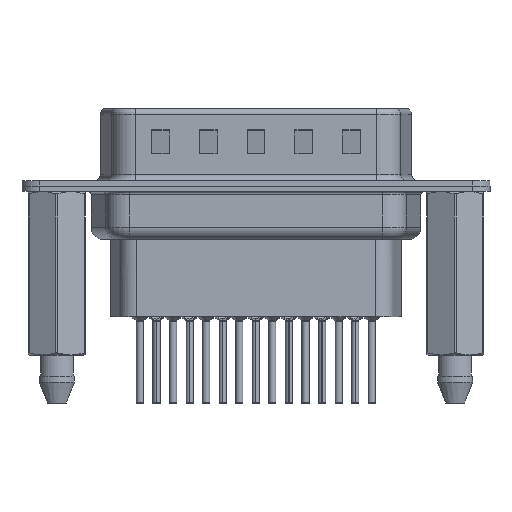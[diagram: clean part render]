
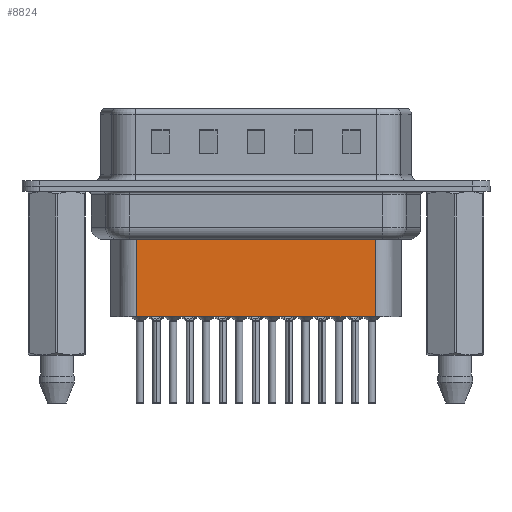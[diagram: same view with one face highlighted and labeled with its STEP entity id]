
A CAD part, front view. The second image highlights one B-rep face of the part: STEP entity #8824.
In plain terms, the highlighted planar face has unit normal (0, -1, 0).
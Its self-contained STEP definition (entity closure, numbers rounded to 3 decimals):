
#224 = DIRECTION ( 'NONE',  ( 0., 0., -1. ) ) ;
#335 = VERTEX_POINT ( 'NONE', #12332 ) ;
#342 = CARTESIAN_POINT ( 'NONE',  ( 6.681, -3.5, -4.097 ) ) ;
#855 = CARTESIAN_POINT ( 'NONE',  ( 6.681, -3.5, -10.95 ) ) ;
#2435 = LINE ( 'NONE', #3901, #16455 ) ;
#2647 = CARTESIAN_POINT ( 'NONE',  ( 26.619, -3.5, -3.1 ) ) ;
#3901 = CARTESIAN_POINT ( 'NONE',  ( 6.434, -3.5, -4.097 ) ) ;
#3915 = ORIENTED_EDGE ( 'NONE', *, *, #12971, .F. ) ;
#6051 = CARTESIAN_POINT ( 'NONE',  ( 6.681, -3.5, -3.1 ) ) ;
#6637 = DIRECTION ( 'NONE',  ( 0., 0., -1. ) ) ;
#8042 = EDGE_CURVE ( 'NONE', #335, #11165, #18271, .T. ) ;
#8824 = ADVANCED_FACE ( 'NONE', ( #21276 ), #17373, .T. ) ;
#9242 = VECTOR ( 'NONE', #6637, 1000. ) ;
#10085 = DIRECTION ( 'NONE',  ( 1., 0., 0. ) ) ;
#11165 = VERTEX_POINT ( 'NONE', #855 ) ;
#11650 = EDGE_LOOP ( 'NONE', ( #3915, #18556, #18949, #13959 ) ) ;
#11795 = CARTESIAN_POINT ( 'NONE',  ( 6.681, -3.5, -3.1 ) ) ;
#11917 = DIRECTION ( 'NONE',  ( 0., -1., 0. ) ) ;
#12161 = VECTOR ( 'NONE', #14511, 1000. ) ;
#12332 = CARTESIAN_POINT ( 'NONE',  ( 26.619, -3.5, -10.95 ) ) ;
#12648 = VERTEX_POINT ( 'NONE', #342 ) ;
#12653 = VERTEX_POINT ( 'NONE', #22449 ) ;
#12818 = EDGE_CURVE ( 'NONE', #12648, #11165, #15257, .T. ) ;
#12971 = EDGE_CURVE ( 'NONE', #12653, #335, #22808, .T. ) ;
#13959 = ORIENTED_EDGE ( 'NONE', *, *, #8042, .F. ) ;
#14511 = DIRECTION ( 'NONE',  ( -1., 0., 0. ) ) ;
#15257 = LINE ( 'NONE', #6051, #17782 ) ;
#16455 = VECTOR ( 'NONE', #22830, 1000. ) ;
#17373 = PLANE ( 'NONE',  #21890 ) ;
#17782 = VECTOR ( 'NONE', #224, 1000. ) ;
#18271 = LINE ( 'NONE', #19991, #12161 ) ;
#18556 = ORIENTED_EDGE ( 'NONE', *, *, #21770, .T. ) ;
#18949 = ORIENTED_EDGE ( 'NONE', *, *, #12818, .T. ) ;
#19991 = CARTESIAN_POINT ( 'NONE',  ( 6.681, -3.5, -10.95 ) ) ;
#21276 = FACE_OUTER_BOUND ( 'NONE', #11650, .T. ) ;
#21770 = EDGE_CURVE ( 'NONE', #12653, #12648, #2435, .T. ) ;
#21890 = AXIS2_PLACEMENT_3D ( 'NONE', #11795, #11917, #10085 ) ;
#22449 = CARTESIAN_POINT ( 'NONE',  ( 26.619, -3.5, -4.097 ) ) ;
#22808 = LINE ( 'NONE', #2647, #9242 ) ;
#22830 = DIRECTION ( 'NONE',  ( -1., 0., 0. ) ) ;
